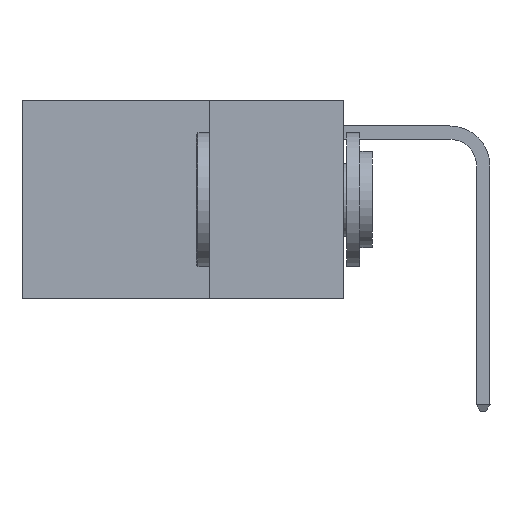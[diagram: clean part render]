
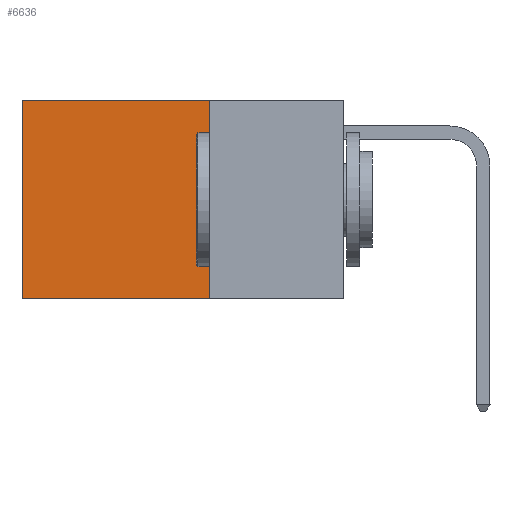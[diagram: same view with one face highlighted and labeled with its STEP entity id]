
A CAD part, left-side view. The second image highlights one B-rep face of the part: STEP entity #6636.
In plain terms, the highlighted planar face has unit normal (-1, 0, 0).
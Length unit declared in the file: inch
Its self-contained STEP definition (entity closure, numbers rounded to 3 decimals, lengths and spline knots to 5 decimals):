
#324 = CARTESIAN_POINT ( 'NONE',  ( 0.2625, 0.6, 0. ) ) ;
#817 = EDGE_CURVE ( 'NONE', #7577, #16944, #10697, .T. ) ;
#1123 = DIRECTION ( 'NONE',  ( 0., 0., -1. ) ) ;
#1167 = FACE_OUTER_BOUND ( 'NONE', #2350, .T. ) ;
#2350 = EDGE_LOOP ( 'NONE', ( #2761, #12794, #17748, #8499 ) ) ;
#2761 = ORIENTED_EDGE ( 'NONE', *, *, #817, .T. ) ;
#3562 = DIRECTION ( 'NONE',  ( 0., 0., -1. ) ) ;
#3646 = LINE ( 'NONE', #6799, #18436 ) ;
#3673 = VERTEX_POINT ( 'NONE', #12602 ) ;
#5427 = PLANE ( 'NONE',  #15279 ) ;
#6636 = ADVANCED_FACE ( 'NONE', ( #1167 ), #5427, .F. ) ;
#6799 = CARTESIAN_POINT ( 'NONE',  ( 0.2625, 0.25, 0. ) ) ;
#6872 = CARTESIAN_POINT ( 'NONE',  ( 0.2625, 0.25, 0. ) ) ;
#7154 = VECTOR ( 'NONE', #3562, 39.37008 ) ;
#7577 = VERTEX_POINT ( 'NONE', #324 ) ;
#7605 = LINE ( 'NONE', #17835, #7154 ) ;
#8250 = DIRECTION ( 'NONE',  ( 0., 1., 0. ) ) ;
#8499 = ORIENTED_EDGE ( 'NONE', *, *, #12814, .T. ) ;
#9742 = DIRECTION ( 'NONE',  ( 1., 0., 0. ) ) ;
#10463 = CARTESIAN_POINT ( 'NONE',  ( 0.2625, 0.25, 0. ) ) ;
#10697 = LINE ( 'NONE', #13069, #18301 ) ;
#11054 = VECTOR ( 'NONE', #17240, 39.37008 ) ;
#12084 = CARTESIAN_POINT ( 'NONE',  ( 0.2625, 0.6, -0.37 ) ) ;
#12602 = CARTESIAN_POINT ( 'NONE',  ( 0.2625, 0.25, -0.37 ) ) ;
#12794 = ORIENTED_EDGE ( 'NONE', *, *, #13015, .F. ) ;
#12814 = EDGE_CURVE ( 'NONE', #18021, #7577, #3646, .T. ) ;
#12910 = CARTESIAN_POINT ( 'NONE',  ( 0.2625, 0.25, -0.37 ) ) ;
#13015 = EDGE_CURVE ( 'NONE', #3673, #16944, #14815, .T. ) ;
#13069 = CARTESIAN_POINT ( 'NONE',  ( 0.2625, 0.6, 0. ) ) ;
#13151 = DIRECTION ( 'NONE',  ( 0., 0., -1. ) ) ;
#14815 = LINE ( 'NONE', #12910, #11054 ) ;
#15279 = AXIS2_PLACEMENT_3D ( 'NONE', #6872, #9742, #1123 ) ;
#16944 = VERTEX_POINT ( 'NONE', #12084 ) ;
#17240 = DIRECTION ( 'NONE',  ( 0., 1., 0. ) ) ;
#17481 = EDGE_CURVE ( 'NONE', #18021, #3673, #7605, .T. ) ;
#17748 = ORIENTED_EDGE ( 'NONE', *, *, #17481, .F. ) ;
#17835 = CARTESIAN_POINT ( 'NONE',  ( 0.2625, 0.25, 0. ) ) ;
#18021 = VERTEX_POINT ( 'NONE', #10463 ) ;
#18301 = VECTOR ( 'NONE', #13151, 39.37008 ) ;
#18436 = VECTOR ( 'NONE', #8250, 39.37008 ) ;
